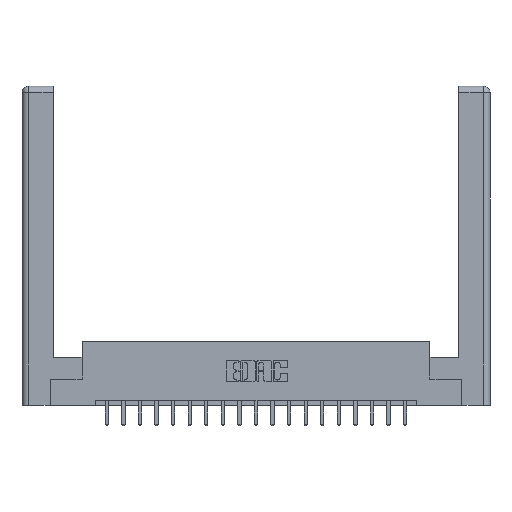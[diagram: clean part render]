
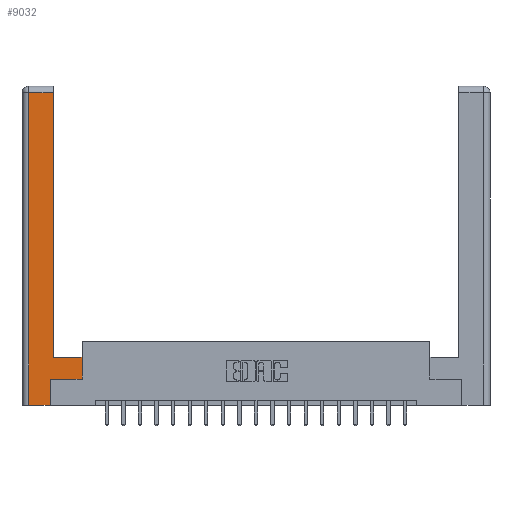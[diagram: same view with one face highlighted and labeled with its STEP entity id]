
A CAD part, top view. The second image highlights one B-rep face of the part: STEP entity #9032.
In plain terms, the highlighted planar face has unit normal (0, 0, 1).
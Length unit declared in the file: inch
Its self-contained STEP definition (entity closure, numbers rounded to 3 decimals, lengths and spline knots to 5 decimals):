
#414 = EDGE_CURVE ( 'NONE', #17787, #1632, #19391, .T. ) ;
#529 = VERTEX_POINT ( 'NONE', #15742 ) ;
#801 = PLANE ( 'NONE',  #6100 ) ;
#870 = DIRECTION ( 'NONE',  ( -1., 0., 0. ) ) ;
#1409 = LINE ( 'NONE', #12539, #16488 ) ;
#1532 = LINE ( 'NONE', #6349, #9398 ) ;
#1632 = VERTEX_POINT ( 'NONE', #3105 ) ;
#1681 = VERTEX_POINT ( 'NONE', #15586 ) ;
#2450 = CARTESIAN_POINT ( 'NONE',  ( 0., 0., 0. ) ) ;
#2566 = EDGE_CURVE ( 'NONE', #19989, #13126, #1532, .T. ) ;
#2951 = FACE_OUTER_BOUND ( 'NONE', #13514, .T. ) ;
#3105 = CARTESIAN_POINT ( 'NONE',  ( 0.265, 0.245, 0. ) ) ;
#3160 = VERTEX_POINT ( 'NONE', #8920 ) ;
#3727 = EDGE_CURVE ( 'NONE', #3160, #12870, #9791, .T. ) ;
#3964 = EDGE_CURVE ( 'NONE', #1632, #529, #16252, .T. ) ;
#3996 = VECTOR ( 'NONE', #9537, 39.37008 ) ;
#4479 = DIRECTION ( 'NONE',  ( -1., 0., 0. ) ) ;
#4565 = ORIENTED_EDGE ( 'NONE', *, *, #3727, .T. ) ;
#4575 = CARTESIAN_POINT ( 'NONE',  ( 0.0615, 0., 0. ) ) ;
#5480 = CARTESIAN_POINT ( 'NONE',  ( 0.295, 0.45, 0. ) ) ;
#5483 = EDGE_CURVE ( 'NONE', #1681, #19989, #1409, .T. ) ;
#6100 = AXIS2_PLACEMENT_3D ( 'NONE', #2450, #11787, #870 ) ;
#6349 = CARTESIAN_POINT ( 'NONE',  ( 0.295, 3., 0. ) ) ;
#6634 = LINE ( 'NONE', #17453, #15572 ) ;
#7294 = CARTESIAN_POINT ( 'NONE',  ( 0.295, 2.94, 0. ) ) ;
#8021 = EDGE_CURVE ( 'NONE', #12870, #17787, #17114, .T. ) ;
#8681 = ORIENTED_EDGE ( 'NONE', *, *, #15325, .T. ) ;
#8920 = CARTESIAN_POINT ( 'NONE',  ( 0.0615, 2.94, 0. ) ) ;
#9032 = ADVANCED_FACE ( 'NONE', ( #2951 ), #801, .F. ) ;
#9250 = CARTESIAN_POINT ( 'NONE',  ( 0.265, 0., 0. ) ) ;
#9398 = VECTOR ( 'NONE', #12416, 39.37008 ) ;
#9537 = DIRECTION ( 'NONE',  ( 1., 0., 0. ) ) ;
#9791 = LINE ( 'NONE', #12070, #14287 ) ;
#10298 = ORIENTED_EDGE ( 'NONE', *, *, #8021, .T. ) ;
#10706 = DIRECTION ( 'NONE',  ( 0., 1., 0. ) ) ;
#11787 = DIRECTION ( 'NONE',  ( 0., 0., -1. ) ) ;
#12070 = CARTESIAN_POINT ( 'NONE',  ( 0.0615, 0., 0. ) ) ;
#12162 = CARTESIAN_POINT ( 'NONE',  ( 0.565, 0.45, 0. ) ) ;
#12415 = VECTOR ( 'NONE', #15672, 39.37008 ) ;
#12416 = DIRECTION ( 'NONE',  ( 0., 1., 0. ) ) ;
#12539 = CARTESIAN_POINT ( 'NONE',  ( 0.295, 0.45, 0. ) ) ;
#12642 = CARTESIAN_POINT ( 'NONE',  ( 0.565, 0.245, 0. ) ) ;
#12870 = VERTEX_POINT ( 'NONE', #4575 ) ;
#12916 = DIRECTION ( 'NONE',  ( -1., 0., 0. ) ) ;
#13126 = VERTEX_POINT ( 'NONE', #7294 ) ;
#13514 = EDGE_LOOP ( 'NONE', ( #19474, #8681, #4565, #10298, #15289, #16401, #17583, #16455 ) ) ;
#13861 = LINE ( 'NONE', #12162, #18838 ) ;
#14287 = VECTOR ( 'NONE', #16613, 39.37008 ) ;
#14351 = CARTESIAN_POINT ( 'NONE',  ( 0.265, 0., 0. ) ) ;
#15289 = ORIENTED_EDGE ( 'NONE', *, *, #414, .T. ) ;
#15325 = EDGE_CURVE ( 'NONE', #13126, #3160, #6634, .T. ) ;
#15572 = VECTOR ( 'NONE', #12916, 39.37008 ) ;
#15586 = CARTESIAN_POINT ( 'NONE',  ( 0.565, 0.45, 0. ) ) ;
#15672 = DIRECTION ( 'NONE',  ( 0., 1., 0. ) ) ;
#15742 = CARTESIAN_POINT ( 'NONE',  ( 0.565, 0.245, 0. ) ) ;
#15953 = DIRECTION ( 'NONE',  ( 1., 0., 0. ) ) ;
#16252 = LINE ( 'NONE', #12642, #17008 ) ;
#16401 = ORIENTED_EDGE ( 'NONE', *, *, #3964, .T. ) ;
#16455 = ORIENTED_EDGE ( 'NONE', *, *, #5483, .T. ) ;
#16488 = VECTOR ( 'NONE', #4479, 39.37008 ) ;
#16613 = DIRECTION ( 'NONE',  ( 0., -1., 0. ) ) ;
#17008 = VECTOR ( 'NONE', #15953, 39.37008 ) ;
#17114 = LINE ( 'NONE', #9250, #3996 ) ;
#17453 = CARTESIAN_POINT ( 'NONE',  ( 0.0615, 2.94, 0. ) ) ;
#17583 = ORIENTED_EDGE ( 'NONE', *, *, #20115, .T. ) ;
#17787 = VERTEX_POINT ( 'NONE', #14351 ) ;
#18838 = VECTOR ( 'NONE', #10706, 39.37008 ) ;
#19391 = LINE ( 'NONE', #20345, #12415 ) ;
#19474 = ORIENTED_EDGE ( 'NONE', *, *, #2566, .T. ) ;
#19989 = VERTEX_POINT ( 'NONE', #5480 ) ;
#20115 = EDGE_CURVE ( 'NONE', #529, #1681, #13861, .T. ) ;
#20345 = CARTESIAN_POINT ( 'NONE',  ( 0.265, 0.245, 0. ) ) ;
